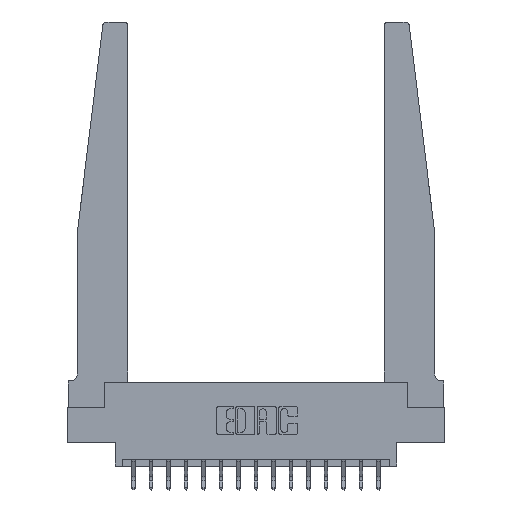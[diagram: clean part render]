
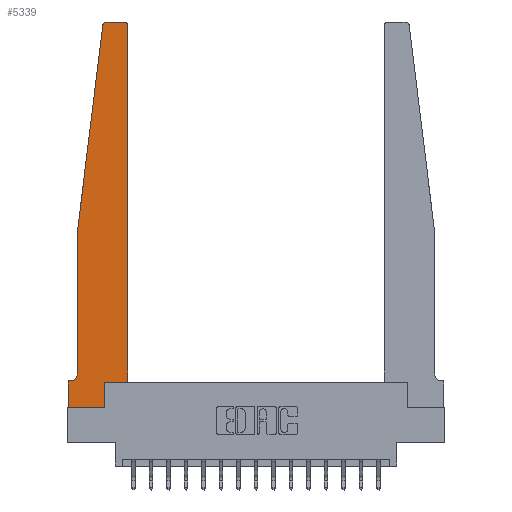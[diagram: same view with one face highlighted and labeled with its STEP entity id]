
A CAD part, top view. The second image highlights one B-rep face of the part: STEP entity #5339.
In plain terms, the highlighted planar face has unit normal (0, 0, 1).
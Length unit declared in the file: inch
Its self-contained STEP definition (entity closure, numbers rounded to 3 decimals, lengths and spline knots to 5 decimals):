
#358 = LINE ( 'NONE', #16574, #10073 ) ;
#685 = CARTESIAN_POINT ( 'NONE',  ( 0.065, 1.25, 0.37 ) ) ;
#728 = EDGE_CURVE ( 'NONE', #10778, #16096, #6486, .T. ) ;
#748 = DIRECTION ( 'NONE',  ( -1., 0., 0. ) ) ;
#855 = ORIENTED_EDGE ( 'NONE', *, *, #4154, .T. ) ;
#1659 = CARTESIAN_POINT ( 'NONE',  ( 0., 0., 0.37 ) ) ;
#1724 = DIRECTION ( 'NONE',  ( 0., 0., -1. ) ) ;
#1770 = CARTESIAN_POINT ( 'NONE',  ( 0.065, 0.2375, 0.37 ) ) ;
#2197 = LINE ( 'NONE', #18516, #16605 ) ;
#2558 = VERTEX_POINT ( 'NONE', #5773 ) ;
#2648 = CARTESIAN_POINT ( 'NONE',  ( 0.2605, 0.18, 0.37 ) ) ;
#2865 = PLANE ( 'NONE',  #18376 ) ;
#2907 = CARTESIAN_POINT ( 'NONE',  ( 0., 0., 0.37 ) ) ;
#3299 = DIRECTION ( 'NONE',  ( 0., 0., 1. ) ) ;
#3315 = EDGE_CURVE ( 'NONE', #5536, #2558, #17979, .T. ) ;
#3585 = ORIENTED_EDGE ( 'NONE', *, *, #6640, .T. ) ;
#3933 = AXIS2_PLACEMENT_3D ( 'NONE', #14864, #1724, #9118 ) ;
#3997 = ORIENTED_EDGE ( 'NONE', *, *, #3315, .T. ) ;
#4065 = CARTESIAN_POINT ( 'NONE',  ( 0.24675, 2.72367, 0.37 ) ) ;
#4154 = EDGE_CURVE ( 'NONE', #13756, #5931, #358, .T. ) ;
#4180 = AXIS2_PLACEMENT_3D ( 'NONE', #16542, #3299, #9262 ) ;
#4313 = ORIENTED_EDGE ( 'NONE', *, *, #5197, .T. ) ;
#4678 = CARTESIAN_POINT ( 'NONE',  ( 0.425, 2.72, 0.37 ) ) ;
#4855 = EDGE_CURVE ( 'NONE', #2558, #6170, #9695, .T. ) ;
#5197 = EDGE_CURVE ( 'NONE', #5931, #7060, #11005, .T. ) ;
#5339 = ADVANCED_FACE ( 'NONE', ( #17352 ), #2865, .T. ) ;
#5387 = DIRECTION ( 'NONE',  ( -0.122, -0.992, 0. ) ) ;
#5536 = VERTEX_POINT ( 'NONE', #4678 ) ;
#5638 = VECTOR ( 'NONE', #15490, 39.37008 ) ;
#5773 = CARTESIAN_POINT ( 'NONE',  ( 0.395, 2.75, 0.37 ) ) ;
#5880 = VERTEX_POINT ( 'NONE', #14640 ) ;
#5931 = VERTEX_POINT ( 'NONE', #1770 ) ;
#6043 = CARTESIAN_POINT ( 'NONE',  ( 0.065, 1.25, 0.37 ) ) ;
#6067 = VECTOR ( 'NONE', #13929, 39.37008 ) ;
#6170 = VERTEX_POINT ( 'NONE', #11166 ) ;
#6456 = VECTOR ( 'NONE', #14283, 39.37008 ) ;
#6486 = LINE ( 'NONE', #9554, #5638 ) ;
#6511 = VECTOR ( 'NONE', #14522, 39.37008 ) ;
#6640 = EDGE_CURVE ( 'NONE', #16096, #5536, #18718, .T. ) ;
#7060 = VERTEX_POINT ( 'NONE', #12729 ) ;
#7209 = CARTESIAN_POINT ( 'NONE',  ( 0.2605, 0.18, 0.37 ) ) ;
#7515 = VERTEX_POINT ( 'NONE', #4065 ) ;
#7516 = LINE ( 'NONE', #1659, #17312 ) ;
#8399 = ORIENTED_EDGE ( 'NONE', *, *, #8893, .T. ) ;
#8893 = EDGE_CURVE ( 'NONE', #7060, #5880, #2197, .T. ) ;
#9118 = DIRECTION ( 'NONE',  ( -1., 0., 0. ) ) ;
#9262 = DIRECTION ( 'NONE',  ( 1., 0., 0. ) ) ;
#9299 = CIRCLE ( 'NONE', #17882, 0.03 ) ;
#9554 = CARTESIAN_POINT ( 'NONE',  ( 0.425, 0.18, 0.37 ) ) ;
#9695 = LINE ( 'NONE', #18443, #6067 ) ;
#9720 = CARTESIAN_POINT ( 'NONE',  ( 0.2605, 0., 0.37 ) ) ;
#9777 = VERTEX_POINT ( 'NONE', #9720 ) ;
#9968 = EDGE_CURVE ( 'NONE', #5880, #14708, #11652, .T. ) ;
#10073 = VECTOR ( 'NONE', #16376, 39.37008 ) ;
#10163 = CARTESIAN_POINT ( 'NONE',  ( 0., 0.1875, 0.37 ) ) ;
#10253 = DIRECTION ( 'NONE',  ( 0., 0., 1. ) ) ;
#10265 = ORIENTED_EDGE ( 'NONE', *, *, #728, .T. ) ;
#10448 = ORIENTED_EDGE ( 'NONE', *, *, #9968, .T. ) ;
#10494 = EDGE_CURVE ( 'NONE', #6170, #7515, #9299, .T. ) ;
#10629 = DIRECTION ( 'NONE',  ( 1., 0., 0. ) ) ;
#10698 = ORIENTED_EDGE ( 'NONE', *, *, #12928, .T. ) ;
#10769 = DIRECTION ( 'NONE',  ( 1., 0., 0. ) ) ;
#10778 = VERTEX_POINT ( 'NONE', #2648 ) ;
#11005 = CIRCLE ( 'NONE', #3933, 0.05 ) ;
#11166 = CARTESIAN_POINT ( 'NONE',  ( 0.27653, 2.75, 0.37 ) ) ;
#11288 = ORIENTED_EDGE ( 'NONE', *, *, #10494, .T. ) ;
#11397 = EDGE_CURVE ( 'NONE', #14708, #9777, #7516, .T. ) ;
#11497 = EDGE_CURVE ( 'NONE', #7515, #13756, #16628, .T. ) ;
#11652 = LINE ( 'NONE', #2907, #6511 ) ;
#11895 = ORIENTED_EDGE ( 'NONE', *, *, #11497, .T. ) ;
#12169 = CARTESIAN_POINT ( 'NONE',  ( 0.27653, 2.72, 0.37 ) ) ;
#12666 = EDGE_LOOP ( 'NONE', ( #13246, #11288, #11895, #855, #4313, #8399, #10448, #18094, #10698, #10265, #3585, #3997 ) ) ;
#12729 = CARTESIAN_POINT ( 'NONE',  ( 0.015, 0.1875, 0.37 ) ) ;
#12928 = EDGE_CURVE ( 'NONE', #9777, #10778, #16031, .T. ) ;
#13246 = ORIENTED_EDGE ( 'NONE', *, *, #4855, .T. ) ;
#13593 = CARTESIAN_POINT ( 'NONE',  ( 0., 0., 0.37 ) ) ;
#13756 = VERTEX_POINT ( 'NONE', #6043 ) ;
#13929 = DIRECTION ( 'NONE',  ( -1., 0., 0. ) ) ;
#14283 = DIRECTION ( 'NONE',  ( 0., 1., 0. ) ) ;
#14440 = VECTOR ( 'NONE', #17461, 39.37008 ) ;
#14522 = DIRECTION ( 'NONE',  ( 0., -1., 0. ) ) ;
#14640 = CARTESIAN_POINT ( 'NONE',  ( 0., 0.1875, 0.37 ) ) ;
#14708 = VERTEX_POINT ( 'NONE', #13593 ) ;
#14844 = DIRECTION ( 'NONE',  ( 0., 0., 1. ) ) ;
#14864 = CARTESIAN_POINT ( 'NONE',  ( 0.015, 0.2375, 0.37 ) ) ;
#15171 = VECTOR ( 'NONE', #5387, 39.37008 ) ;
#15175 = CARTESIAN_POINT ( 'NONE',  ( 0.425, 0.18, 0.37 ) ) ;
#15490 = DIRECTION ( 'NONE',  ( 1., 0., 0. ) ) ;
#15912 = DIRECTION ( 'NONE',  ( 1., 0., 0. ) ) ;
#16031 = LINE ( 'NONE', #7209, #14440 ) ;
#16096 = VERTEX_POINT ( 'NONE', #17982 ) ;
#16376 = DIRECTION ( 'NONE',  ( 0., -1., 0. ) ) ;
#16542 = CARTESIAN_POINT ( 'NONE',  ( 0.395, 2.72, 0.37 ) ) ;
#16574 = CARTESIAN_POINT ( 'NONE',  ( 0.065, 1.25, 0.37 ) ) ;
#16605 = VECTOR ( 'NONE', #748, 39.37008 ) ;
#16628 = LINE ( 'NONE', #685, #15171 ) ;
#17312 = VECTOR ( 'NONE', #10769, 39.37008 ) ;
#17352 = FACE_OUTER_BOUND ( 'NONE', #12666, .T. ) ;
#17461 = DIRECTION ( 'NONE',  ( 0., 1., 0. ) ) ;
#17882 = AXIS2_PLACEMENT_3D ( 'NONE', #12169, #14844, #10629 ) ;
#17979 = CIRCLE ( 'NONE', #4180, 0.03 ) ;
#17982 = CARTESIAN_POINT ( 'NONE',  ( 0.425, 0.18, 0.37 ) ) ;
#18094 = ORIENTED_EDGE ( 'NONE', *, *, #11397, .T. ) ;
#18376 = AXIS2_PLACEMENT_3D ( 'NONE', #10163, #10253, #15912 ) ;
#18443 = CARTESIAN_POINT ( 'NONE',  ( 0.25, 2.75, 0.37 ) ) ;
#18516 = CARTESIAN_POINT ( 'NONE',  ( 0.065, 0.1875, 0.37 ) ) ;
#18718 = LINE ( 'NONE', #15175, #6456 ) ;
